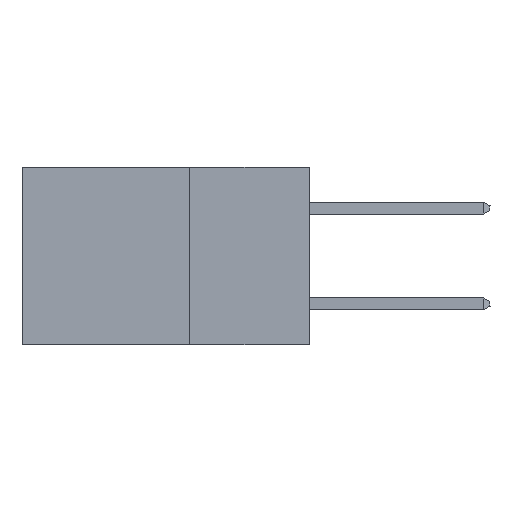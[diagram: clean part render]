
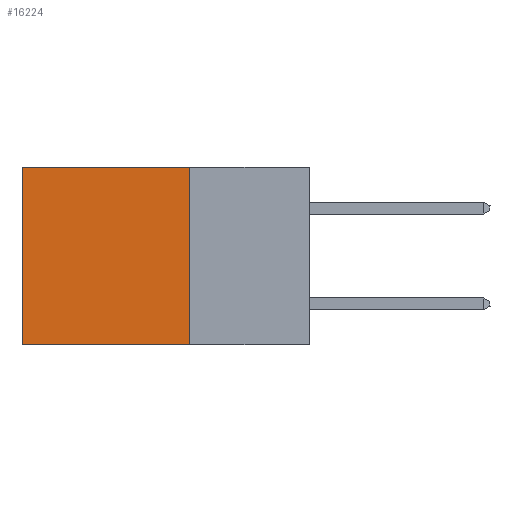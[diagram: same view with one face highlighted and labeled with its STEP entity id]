
A CAD part, left-side view. The second image highlights one B-rep face of the part: STEP entity #16224.
In plain terms, the highlighted planar face has unit normal (-1, 0, 0).
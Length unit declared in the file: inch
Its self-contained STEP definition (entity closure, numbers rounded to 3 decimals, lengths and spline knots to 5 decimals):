
#697 = CARTESIAN_POINT ( 'NONE',  ( 0.2875, 0.25, 0. ) ) ;
#1106 = VECTOR ( 'NONE', #14926, 39.37008 ) ;
#1843 = DIRECTION ( 'NONE',  ( 0., 0., -1. ) ) ;
#1940 = DIRECTION ( 'NONE',  ( 1., 0., 0. ) ) ;
#2313 = CARTESIAN_POINT ( 'NONE',  ( 0.2875, 0.6, -0.37 ) ) ;
#8157 = EDGE_CURVE ( 'NONE', #8461, #14791, #19982, .T. ) ;
#8461 = VERTEX_POINT ( 'NONE', #20222 ) ;
#8864 = PLANE ( 'NONE',  #33624 ) ;
#9556 = EDGE_CURVE ( 'NONE', #14791, #29030, #24676, .T. ) ;
#9696 = LINE ( 'NONE', #20900, #41960 ) ;
#13456 = ORIENTED_EDGE ( 'NONE', *, *, #8157, .T. ) ;
#13625 = CARTESIAN_POINT ( 'NONE',  ( 0.2875, 0.25, -0.37 ) ) ;
#14791 = VERTEX_POINT ( 'NONE', #22177 ) ;
#14926 = DIRECTION ( 'NONE',  ( 0., 1., 0. ) ) ;
#15238 = VECTOR ( 'NONE', #1843, 39.37008 ) ;
#16224 = ADVANCED_FACE ( 'NONE', ( #18368 ), #8864, .F. ) ;
#18368 = FACE_OUTER_BOUND ( 'NONE', #37531, .T. ) ;
#19925 = EDGE_CURVE ( 'NONE', #37322, #29030, #38109, .T. ) ;
#19982 = LINE ( 'NONE', #697, #1106 ) ;
#20222 = CARTESIAN_POINT ( 'NONE',  ( 0.2875, 0.25, 0. ) ) ;
#20510 = EDGE_CURVE ( 'NONE', #8461, #37322, #9696, .T. ) ;
#20900 = CARTESIAN_POINT ( 'NONE',  ( 0.2875, 0.25, 0. ) ) ;
#22177 = CARTESIAN_POINT ( 'NONE',  ( 0.2875, 0.6, 0. ) ) ;
#24676 = LINE ( 'NONE', #26648, #15238 ) ;
#26648 = CARTESIAN_POINT ( 'NONE',  ( 0.2875, 0.6, 0. ) ) ;
#26745 = DIRECTION ( 'NONE',  ( 0., 0., -1. ) ) ;
#29030 = VERTEX_POINT ( 'NONE', #2313 ) ;
#29778 = VECTOR ( 'NONE', #38491, 39.37008 ) ;
#33624 = AXIS2_PLACEMENT_3D ( 'NONE', #37311, #1940, #26745 ) ;
#37311 = CARTESIAN_POINT ( 'NONE',  ( 0.2875, 0.25, 0. ) ) ;
#37322 = VERTEX_POINT ( 'NONE', #39101 ) ;
#37531 = EDGE_LOOP ( 'NONE', ( #40828, #38704, #40409, #13456 ) ) ;
#38109 = LINE ( 'NONE', #13625, #29778 ) ;
#38491 = DIRECTION ( 'NONE',  ( 0., 1., 0. ) ) ;
#38704 = ORIENTED_EDGE ( 'NONE', *, *, #19925, .F. ) ;
#39101 = CARTESIAN_POINT ( 'NONE',  ( 0.2875, 0.25, -0.37 ) ) ;
#40409 = ORIENTED_EDGE ( 'NONE', *, *, #20510, .F. ) ;
#40828 = ORIENTED_EDGE ( 'NONE', *, *, #9556, .T. ) ;
#41960 = VECTOR ( 'NONE', #42180, 39.37008 ) ;
#42180 = DIRECTION ( 'NONE',  ( 0., 0., -1. ) ) ;
